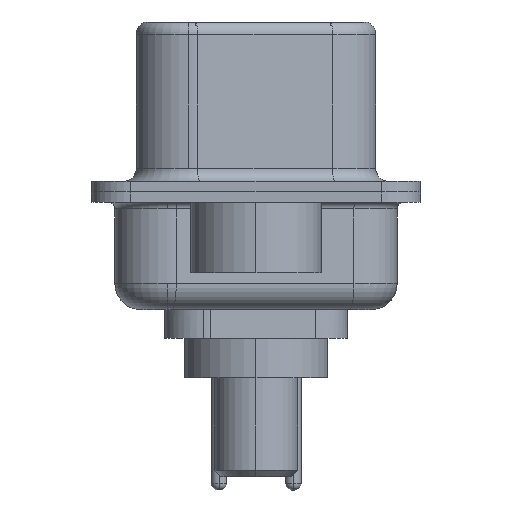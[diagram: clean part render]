
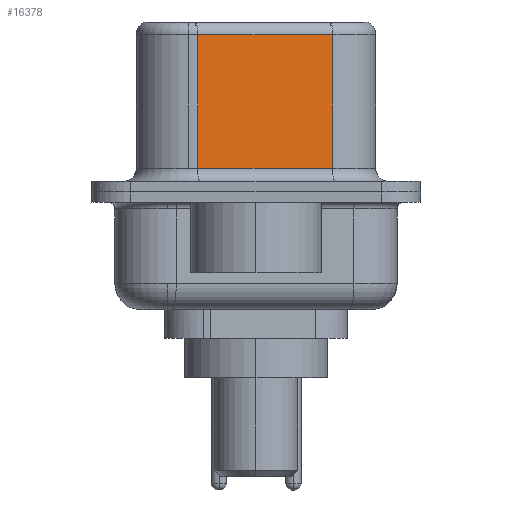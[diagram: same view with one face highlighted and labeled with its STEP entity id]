
A CAD part, left-side view. The second image highlights one B-rep face of the part: STEP entity #16378.
In plain terms, the highlighted planar face has unit normal (-0.985, -0.174, 0).
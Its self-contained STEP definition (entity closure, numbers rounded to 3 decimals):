
#1780 = VERTEX_POINT ( 'NONE', #20647 ) ;
#2105 = CARTESIAN_POINT ( 'NONE',  ( 4.58, -2.927, 0.9 ) ) ;
#2451 = AXIS2_PLACEMENT_3D ( 'NONE', #10891, #9041, #22783 ) ;
#2749 = VERTEX_POINT ( 'NONE', #19981 ) ;
#3478 = EDGE_CURVE ( 'NONE', #2749, #24239, #16881, .T. ) ;
#4536 = ORIENTED_EDGE ( 'NONE', *, *, #11926, .T. ) ;
#5375 = VERTEX_POINT ( 'NONE', #8677 ) ;
#6127 = EDGE_CURVE ( 'NONE', #2749, #1780, #8674, .T. ) ;
#6265 = CARTESIAN_POINT ( 'NONE',  ( 4.58, -2.927, 0.9 ) ) ;
#6670 = EDGE_CURVE ( 'NONE', #1780, #5375, #24962, .T. ) ;
#7460 = VECTOR ( 'NONE', #7461, 1000. ) ;
#7461 = DIRECTION ( 'NONE',  ( -0.174, 0.985, 0. ) ) ;
#8674 = LINE ( 'NONE', #17251, #7460 ) ;
#8677 = CARTESIAN_POINT ( 'NONE',  ( 3.67, 2.233, 0.9 ) ) ;
#8866 = DIRECTION ( 'NONE',  ( 0., 0., -1. ) ) ;
#9041 = DIRECTION ( 'NONE',  ( 0.985, 0.174, 0. ) ) ;
#9264 = VECTOR ( 'NONE', #8866, 1000. ) ;
#10891 = CARTESIAN_POINT ( 'NONE',  ( 4.58, -2.927, 6.52 ) ) ;
#11704 = VECTOR ( 'NONE', #19221, 1000. ) ;
#11926 = EDGE_CURVE ( 'NONE', #5375, #24239, #22141, .T. ) ;
#14463 = FACE_OUTER_BOUND ( 'NONE', #19137, .T. ) ;
#15818 = DIRECTION ( 'NONE',  ( 0.174, -0.985, 0. ) ) ;
#16378 = ADVANCED_FACE ( 'NONE', ( #14463 ), #16871, .F. ) ;
#16871 = PLANE ( 'NONE',  #2451 ) ;
#16881 = LINE ( 'NONE', #17187, #11704 ) ;
#17187 = CARTESIAN_POINT ( 'NONE',  ( 4.58, -2.927, 6.52 ) ) ;
#17251 = CARTESIAN_POINT ( 'NONE',  ( 4.58, -2.927, 6.02 ) ) ;
#17546 = VECTOR ( 'NONE', #15818, 1000. ) ;
#19137 = EDGE_LOOP ( 'NONE', ( #23809, #23290, #23687, #4536 ) ) ;
#19221 = DIRECTION ( 'NONE',  ( 0., 0., -1. ) ) ;
#19981 = CARTESIAN_POINT ( 'NONE',  ( 4.58, -2.927, 6.02 ) ) ;
#20630 = CARTESIAN_POINT ( 'NONE',  ( 3.67, 2.233, 6.52 ) ) ;
#20647 = CARTESIAN_POINT ( 'NONE',  ( 3.67, 2.233, 6.02 ) ) ;
#22141 = LINE ( 'NONE', #2105, #17546 ) ;
#22783 = DIRECTION ( 'NONE',  ( -0.174, 0.985, 0. ) ) ;
#23290 = ORIENTED_EDGE ( 'NONE', *, *, #6127, .T. ) ;
#23687 = ORIENTED_EDGE ( 'NONE', *, *, #6670, .T. ) ;
#23809 = ORIENTED_EDGE ( 'NONE', *, *, #3478, .F. ) ;
#24239 = VERTEX_POINT ( 'NONE', #6265 ) ;
#24962 = LINE ( 'NONE', #20630, #9264 ) ;
